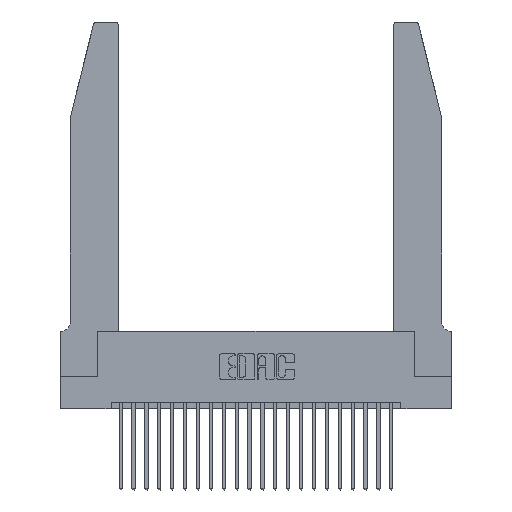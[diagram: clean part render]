
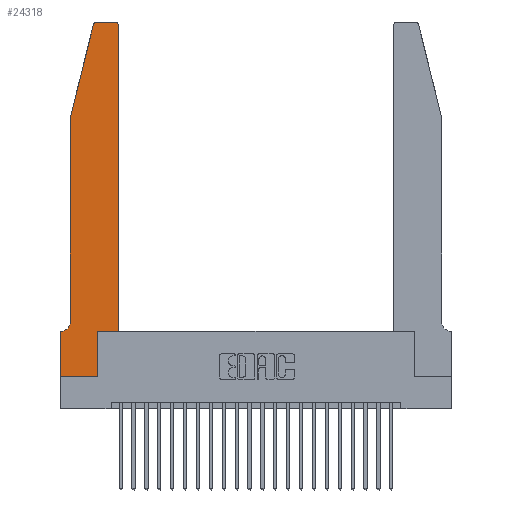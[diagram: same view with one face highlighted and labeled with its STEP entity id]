
A CAD part, top view. The second image highlights one B-rep face of the part: STEP entity #24318.
In plain terms, the highlighted planar face has unit normal (0, 0, 1).
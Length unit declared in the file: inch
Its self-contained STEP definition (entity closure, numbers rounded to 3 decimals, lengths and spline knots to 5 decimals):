
#1047 = ORIENTED_EDGE ( 'NONE', *, *, #20900, .T. ) ;
#1113 = ORIENTED_EDGE ( 'NONE', *, *, #19192, .T. ) ;
#1122 = ORIENTED_EDGE ( 'NONE', *, *, #16497, .T. ) ;
#1286 = DIRECTION ( 'NONE',  ( 0., 0., -1. ) ) ;
#1296 = CARTESIAN_POINT ( 'NONE',  ( 0.0055, 0.35, 0.37 ) ) ;
#1380 = VERTEX_POINT ( 'NONE', #5583 ) ;
#1438 = EDGE_CURVE ( 'NONE', #5756, #18989, #22577, .T. ) ;
#1489 = AXIS2_PLACEMENT_3D ( 'NONE', #8227, #21515, #10191 ) ;
#2202 = DIRECTION ( 'NONE',  ( -1., 0., 0. ) ) ;
#2310 = VECTOR ( 'NONE', #3169, 39.37008 ) ;
#2590 = CARTESIAN_POINT ( 'NONE',  ( 0.0755, 0.35, 0.37 ) ) ;
#2668 = FACE_OUTER_BOUND ( 'NONE', #5925, .T. ) ;
#2895 = EDGE_CURVE ( 'NONE', #4680, #23984, #8294, .T. ) ;
#2937 = VECTOR ( 'NONE', #11675, 39.37008 ) ;
#3169 = DIRECTION ( 'NONE',  ( 0., 1., 0. ) ) ;
#3255 = CARTESIAN_POINT ( 'NONE',  ( 0.0055, 0.42, 0.37 ) ) ;
#3293 = ORIENTED_EDGE ( 'NONE', *, *, #19893, .T. ) ;
#4678 = ORIENTED_EDGE ( 'NONE', *, *, #9697, .T. ) ;
#4680 = VERTEX_POINT ( 'NONE', #22896 ) ;
#4804 = ORIENTED_EDGE ( 'NONE', *, *, #8868, .T. ) ;
#4892 = AXIS2_PLACEMENT_3D ( 'NONE', #3255, #1286, #2202 ) ;
#4913 = CARTESIAN_POINT ( 'NONE',  ( 0.4505, 2.72, 0.37 ) ) ;
#4950 = AXIS2_PLACEMENT_3D ( 'NONE', #19665, #8202, #21498 ) ;
#5146 = ORIENTED_EDGE ( 'NONE', *, *, #1438, .T. ) ;
#5396 = EDGE_CURVE ( 'NONE', #18826, #10786, #12984, .T. ) ;
#5523 = ORIENTED_EDGE ( 'NONE', *, *, #22259, .T. ) ;
#5583 = CARTESIAN_POINT ( 'NONE',  ( 0.2865, 0.35, 0.37 ) ) ;
#5618 = CARTESIAN_POINT ( 'NONE',  ( 0., 0., 0.37 ) ) ;
#5756 = VERTEX_POINT ( 'NONE', #10797 ) ;
#5819 = CARTESIAN_POINT ( 'NONE',  ( 0.2605, 2.75, 0.37 ) ) ;
#5925 = EDGE_LOOP ( 'NONE', ( #14312, #14053, #15029, #4678, #5146, #4804, #1047, #11766, #1113, #1122, #3293, #5523 ) ) ;
#6278 = VERTEX_POINT ( 'NONE', #12308 ) ;
#6298 = VECTOR ( 'NONE', #24403, 39.37008 ) ;
#8202 = DIRECTION ( 'NONE',  ( 0., 0., 1. ) ) ;
#8227 = CARTESIAN_POINT ( 'NONE',  ( 0., 0.35, 0.37 ) ) ;
#8294 = LINE ( 'NONE', #13582, #21663 ) ;
#8404 = VECTOR ( 'NONE', #16140, 39.37008 ) ;
#8868 = EDGE_CURVE ( 'NONE', #18989, #6278, #18038, .T. ) ;
#9188 = AXIS2_PLACEMENT_3D ( 'NONE', #21722, #10388, #23561 ) ;
#9511 = CARTESIAN_POINT ( 'NONE',  ( 0.2865, 0., 0.37 ) ) ;
#9697 = EDGE_CURVE ( 'NONE', #23984, #5756, #11417, .T. ) ;
#10191 = DIRECTION ( 'NONE',  ( 1., 0., 0. ) ) ;
#10262 = VERTEX_POINT ( 'NONE', #14749 ) ;
#10388 = DIRECTION ( 'NONE',  ( 0., 0., 1. ) ) ;
#10786 = VERTEX_POINT ( 'NONE', #16132 ) ;
#10797 = CARTESIAN_POINT ( 'NONE',  ( 0.0755, 0.42, 0.37 ) ) ;
#10888 = DIRECTION ( 'NONE',  ( 1., 0., 0. ) ) ;
#10903 = VERTEX_POINT ( 'NONE', #4913 ) ;
#11284 = CARTESIAN_POINT ( 'NONE',  ( 0.0755, 2., 0.37 ) ) ;
#11417 = LINE ( 'NONE', #11284, #6298 ) ;
#11496 = EDGE_CURVE ( 'NONE', #10262, #12723, #18795, .T. ) ;
#11675 = DIRECTION ( 'NONE',  ( 0., 1., 0. ) ) ;
#11766 = ORIENTED_EDGE ( 'NONE', *, *, #11496, .T. ) ;
#12308 = CARTESIAN_POINT ( 'NONE',  ( 0., 0.35, 0.37 ) ) ;
#12604 = CIRCLE ( 'NONE', #9188, 0.03 ) ;
#12723 = VERTEX_POINT ( 'NONE', #9511 ) ;
#12837 = CARTESIAN_POINT ( 'NONE',  ( 0.4505, 0.35, 0.37 ) ) ;
#12984 = LINE ( 'NONE', #5819, #22925 ) ;
#13151 = VECTOR ( 'NONE', #17609, 39.37008 ) ;
#13272 = LINE ( 'NONE', #12837, #2310 ) ;
#13582 = CARTESIAN_POINT ( 'NONE',  ( 0.0755, 2., 0.37 ) ) ;
#13962 = EDGE_CURVE ( 'NONE', #10786, #4680, #12604, .T. ) ;
#14053 = ORIENTED_EDGE ( 'NONE', *, *, #13962, .T. ) ;
#14312 = ORIENTED_EDGE ( 'NONE', *, *, #5396, .T. ) ;
#14328 = CARTESIAN_POINT ( 'NONE',  ( 0.4205, 2.75, 0.37 ) ) ;
#14749 = CARTESIAN_POINT ( 'NONE',  ( 0., 0., 0.37 ) ) ;
#15029 = ORIENTED_EDGE ( 'NONE', *, *, #2895, .T. ) ;
#15236 = DIRECTION ( 'NONE',  ( 1., 0., 0. ) ) ;
#15741 = CARTESIAN_POINT ( 'NONE',  ( 0., 0., 0.37 ) ) ;
#16132 = CARTESIAN_POINT ( 'NONE',  ( 0.284, 2.75, 0.37 ) ) ;
#16140 = DIRECTION ( 'NONE',  ( -1., 0., 0. ) ) ;
#16497 = EDGE_CURVE ( 'NONE', #1380, #19311, #21583, .T. ) ;
#17315 = DIRECTION ( 'NONE',  ( -1., 0., 0. ) ) ;
#17585 = LINE ( 'NONE', #15741, #13151 ) ;
#17609 = DIRECTION ( 'NONE',  ( 0., -1., 0. ) ) ;
#17707 = LINE ( 'NONE', #19928, #2937 ) ;
#17847 = CARTESIAN_POINT ( 'NONE',  ( 0.4505, 0.35, 0.37 ) ) ;
#18038 = LINE ( 'NONE', #2590, #8404 ) ;
#18203 = VECTOR ( 'NONE', #15236, 39.37008 ) ;
#18795 = LINE ( 'NONE', #5618, #18203 ) ;
#18826 = VERTEX_POINT ( 'NONE', #14328 ) ;
#18989 = VERTEX_POINT ( 'NONE', #1296 ) ;
#19192 = EDGE_CURVE ( 'NONE', #12723, #1380, #17707, .T. ) ;
#19267 = DIRECTION ( 'NONE',  ( -0.239, -0.971, 0. ) ) ;
#19311 = VERTEX_POINT ( 'NONE', #17847 ) ;
#19665 = CARTESIAN_POINT ( 'NONE',  ( 0.4205, 2.72, 0.37 ) ) ;
#19687 = PLANE ( 'NONE',  #1489 ) ;
#19893 = EDGE_CURVE ( 'NONE', #19311, #10903, #13272, .T. ) ;
#19928 = CARTESIAN_POINT ( 'NONE',  ( 0.2865, 0.35, 0.37 ) ) ;
#20345 = CARTESIAN_POINT ( 'NONE',  ( 0.4505, 0.35, 0.37 ) ) ;
#20900 = EDGE_CURVE ( 'NONE', #6278, #10262, #17585, .T. ) ;
#21005 = VECTOR ( 'NONE', #10888, 39.37008 ) ;
#21498 = DIRECTION ( 'NONE',  ( 1., 0., 0. ) ) ;
#21515 = DIRECTION ( 'NONE',  ( 0., 0., 1. ) ) ;
#21583 = LINE ( 'NONE', #20345, #21005 ) ;
#21663 = VECTOR ( 'NONE', #19267, 39.37008 ) ;
#21722 = CARTESIAN_POINT ( 'NONE',  ( 0.284, 2.72, 0.37 ) ) ;
#22259 = EDGE_CURVE ( 'NONE', #10903, #18826, #23899, .T. ) ;
#22577 = CIRCLE ( 'NONE', #4892, 0.07 ) ;
#22896 = CARTESIAN_POINT ( 'NONE',  ( 0.25487, 2.72718, 0.37 ) ) ;
#22925 = VECTOR ( 'NONE', #17315, 39.37008 ) ;
#23561 = DIRECTION ( 'NONE',  ( 1., 0., 0. ) ) ;
#23899 = CIRCLE ( 'NONE', #4950, 0.03 ) ;
#23984 = VERTEX_POINT ( 'NONE', #24110 ) ;
#24110 = CARTESIAN_POINT ( 'NONE',  ( 0.0755, 2., 0.37 ) ) ;
#24318 = ADVANCED_FACE ( 'NONE', ( #2668 ), #19687, .T. ) ;
#24403 = DIRECTION ( 'NONE',  ( 0., -1., 0. ) ) ;
